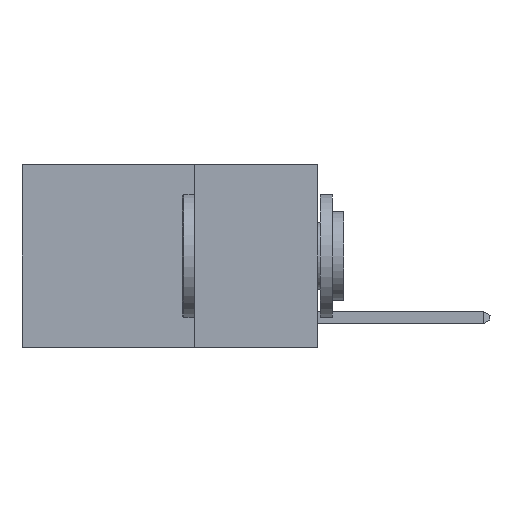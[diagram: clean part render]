
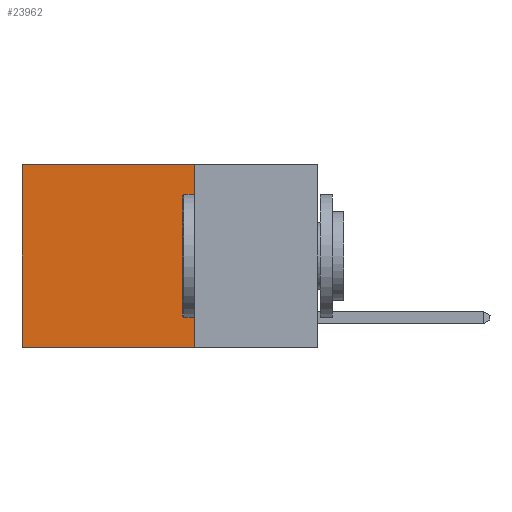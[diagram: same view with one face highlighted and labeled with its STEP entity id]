
A CAD part, left-side view. The second image highlights one B-rep face of the part: STEP entity #23962.
In plain terms, the highlighted planar face has unit normal (-1, 0, 0).
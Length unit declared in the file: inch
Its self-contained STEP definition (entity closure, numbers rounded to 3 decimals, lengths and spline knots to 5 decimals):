
#11 = DIRECTION ( 'NONE',  ( 0., 1., 0. ) ) ;
#1242 = VECTOR ( 'NONE', #18122, 39.37008 ) ;
#1265 = CARTESIAN_POINT ( 'NONE',  ( 0.2625, 0.25, 0. ) ) ;
#1865 = DIRECTION ( 'NONE',  ( 0., 0., -1. ) ) ;
#3981 = CARTESIAN_POINT ( 'NONE',  ( 0.2625, 0.6, -0.37 ) ) ;
#4446 = EDGE_CURVE ( 'NONE', #17776, #8006, #10774, .T. ) ;
#4815 = CARTESIAN_POINT ( 'NONE',  ( 0.2625, 0.6, 0. ) ) ;
#5036 = CARTESIAN_POINT ( 'NONE',  ( 0.2625, 0.25, -0.37 ) ) ;
#5793 = ORIENTED_EDGE ( 'NONE', *, *, #12958, .F. ) ;
#5883 = VECTOR ( 'NONE', #6922, 39.37008 ) ;
#6509 = ORIENTED_EDGE ( 'NONE', *, *, #11245, .F. ) ;
#6922 = DIRECTION ( 'NONE',  ( 0., 0., -1. ) ) ;
#7759 = VERTEX_POINT ( 'NONE', #1265 ) ;
#8006 = VERTEX_POINT ( 'NONE', #3981 ) ;
#9536 = CARTESIAN_POINT ( 'NONE',  ( 0.2625, 0.25, 0. ) ) ;
#9975 = VECTOR ( 'NONE', #11, 39.37008 ) ;
#10224 = CARTESIAN_POINT ( 'NONE',  ( 0.2625, 0.25, -0.37 ) ) ;
#10774 = LINE ( 'NONE', #24162, #20645 ) ;
#11245 = EDGE_CURVE ( 'NONE', #7759, #16406, #20746, .T. ) ;
#11376 = LINE ( 'NONE', #5036, #1242 ) ;
#11498 = EDGE_CURVE ( 'NONE', #7759, #17776, #14940, .T. ) ;
#12958 = EDGE_CURVE ( 'NONE', #16406, #8006, #11376, .T. ) ;
#13091 = DIRECTION ( 'NONE',  ( 0., 0., -1. ) ) ;
#13231 = DIRECTION ( 'NONE',  ( 1., 0., 0. ) ) ;
#14389 = CARTESIAN_POINT ( 'NONE',  ( 0.2625, 0.25, 0. ) ) ;
#14940 = LINE ( 'NONE', #9536, #9975 ) ;
#16406 = VERTEX_POINT ( 'NONE', #10224 ) ;
#17776 = VERTEX_POINT ( 'NONE', #4815 ) ;
#18122 = DIRECTION ( 'NONE',  ( 0., 1., 0. ) ) ;
#20645 = VECTOR ( 'NONE', #13091, 39.37008 ) ;
#20746 = LINE ( 'NONE', #14389, #5883 ) ;
#20949 = AXIS2_PLACEMENT_3D ( 'NONE', #24304, #13231, #1865 ) ;
#21957 = EDGE_LOOP ( 'NONE', ( #23481, #5793, #6509, #22922 ) ) ;
#22470 = PLANE ( 'NONE',  #20949 ) ;
#22922 = ORIENTED_EDGE ( 'NONE', *, *, #11498, .T. ) ;
#23092 = FACE_OUTER_BOUND ( 'NONE', #21957, .T. ) ;
#23481 = ORIENTED_EDGE ( 'NONE', *, *, #4446, .T. ) ;
#23962 = ADVANCED_FACE ( 'NONE', ( #23092 ), #22470, .F. ) ;
#24162 = CARTESIAN_POINT ( 'NONE',  ( 0.2625, 0.6, 0. ) ) ;
#24304 = CARTESIAN_POINT ( 'NONE',  ( 0.2625, 0.25, 0. ) ) ;
